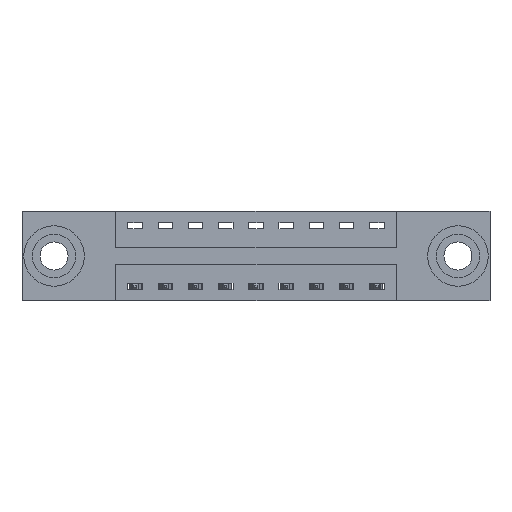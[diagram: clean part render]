
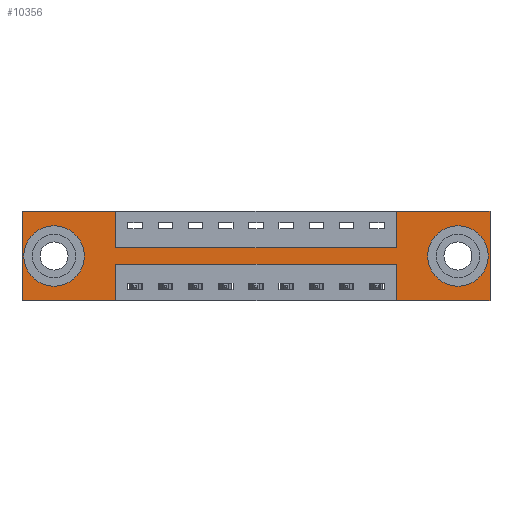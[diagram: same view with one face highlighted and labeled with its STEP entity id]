
A CAD part, front view. The second image highlights one B-rep face of the part: STEP entity #10356.
In plain terms, the highlighted planar face has unit normal (0, -1, 0).
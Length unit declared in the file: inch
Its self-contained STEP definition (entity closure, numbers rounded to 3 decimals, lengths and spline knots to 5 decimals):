
#183 = VERTEX_POINT ( 'NONE', #690 ) ;
#294 = DIRECTION ( 'NONE',  ( 0., -1., 0. ) ) ;
#352 = ORIENTED_EDGE ( 'NONE', *, *, #1826, .F. ) ;
#356 = CARTESIAN_POINT ( 'NONE',  ( 0.3875, 0., -0.22 ) ) ;
#470 = VERTEX_POINT ( 'NONE', #2785 ) ;
#529 = EDGE_CURVE ( 'NONE', #183, #3488, #4031, .T. ) ;
#548 = VECTOR ( 'NONE', #10347, 39.37008 ) ;
#568 = DIRECTION ( 'NONE',  ( 0., 0., -1. ) ) ;
#613 = DIRECTION ( 'NONE',  ( 0., 1., 0. ) ) ;
#633 = VECTOR ( 'NONE', #4701, 39.37008 ) ;
#659 = ORIENTED_EDGE ( 'NONE', *, *, #9545, .F. ) ;
#690 = CARTESIAN_POINT ( 'NONE',  ( 0., 0., -0.37 ) ) ;
#756 = ORIENTED_EDGE ( 'NONE', *, *, #10024, .T. ) ;
#826 = CARTESIAN_POINT ( 'NONE',  ( 0.3875, 0., -0.37 ) ) ;
#841 = LINE ( 'NONE', #9547, #9403 ) ;
#1276 = EDGE_LOOP ( 'NONE', ( #756, #8904 ) ) ;
#1315 = ORIENTED_EDGE ( 'NONE', *, *, #1736, .F. ) ;
#1346 = EDGE_CURVE ( 'NONE', #7675, #6904, #7158, .T. ) ;
#1589 = EDGE_CURVE ( 'NONE', #7468, #2087, #6758, .T. ) ;
#1601 = EDGE_CURVE ( 'NONE', #6904, #7675, #2371, .T. ) ;
#1736 = EDGE_CURVE ( 'NONE', #4805, #8246, #5458, .T. ) ;
#1826 = EDGE_CURVE ( 'NONE', #7963, #7468, #4422, .T. ) ;
#1853 = VERTEX_POINT ( 'NONE', #5337 ) ;
#1908 = FACE_OUTER_BOUND ( 'NONE', #7439, .T. ) ;
#1966 = EDGE_CURVE ( 'NONE', #9443, #183, #4812, .T. ) ;
#2033 = CARTESIAN_POINT ( 'NONE',  ( 0., 0., 0. ) ) ;
#2086 = AXIS2_PLACEMENT_3D ( 'NONE', #5556, #613, #6384 ) ;
#2087 = VERTEX_POINT ( 'NONE', #2345 ) ;
#2157 = ORIENTED_EDGE ( 'NONE', *, *, #1601, .T. ) ;
#2175 = FACE_BOUND ( 'NONE', #1276, .T. ) ;
#2242 = DIRECTION ( 'NONE',  ( 0., 1., 0. ) ) ;
#2345 = CARTESIAN_POINT ( 'NONE',  ( 1.5475, 0., -0.15 ) ) ;
#2371 = CIRCLE ( 'NONE', #2840, 0.078 ) ;
#2435 = ORIENTED_EDGE ( 'NONE', *, *, #1966, .F. ) ;
#2446 = ORIENTED_EDGE ( 'NONE', *, *, #3719, .F. ) ;
#2453 = CIRCLE ( 'NONE', #2086, 0.078 ) ;
#2479 = VECTOR ( 'NONE', #2958, 39.37008 ) ;
#2575 = LINE ( 'NONE', #9696, #633 ) ;
#2686 = DIRECTION ( 'NONE',  ( -1., 0., 0. ) ) ;
#2741 = LINE ( 'NONE', #2033, #548 ) ;
#2785 = CARTESIAN_POINT ( 'NONE',  ( 0.1325, 0., -0.107 ) ) ;
#2794 = ORIENTED_EDGE ( 'NONE', *, *, #1346, .T. ) ;
#2839 = CIRCLE ( 'NONE', #4439, 0.078 ) ;
#2840 = AXIS2_PLACEMENT_3D ( 'NONE', #8331, #3364, #9162 ) ;
#2868 = CARTESIAN_POINT ( 'NONE',  ( 0.3875, 0., -0.37 ) ) ;
#2958 = DIRECTION ( 'NONE',  ( 0., 0., 1. ) ) ;
#3050 = AXIS2_PLACEMENT_3D ( 'NONE', #10497, #5500, #568 ) ;
#3111 = VECTOR ( 'NONE', #4942, 39.37008 ) ;
#3279 = EDGE_CURVE ( 'NONE', #8254, #9443, #3356, .T. ) ;
#3356 = LINE ( 'NONE', #826, #3111 ) ;
#3364 = DIRECTION ( 'NONE',  ( 0., 1., 0. ) ) ;
#3365 = EDGE_LOOP ( 'NONE', ( #2794, #2157 ) ) ;
#3488 = VERTEX_POINT ( 'NONE', #6886 ) ;
#3719 = EDGE_CURVE ( 'NONE', #8246, #10174, #2575, .T. ) ;
#3782 = CARTESIAN_POINT ( 'NONE',  ( 0.3875, 0., -0.22 ) ) ;
#3908 = DIRECTION ( 'NONE',  ( 1., 0., 0. ) ) ;
#4031 = LINE ( 'NONE', #5329, #5977 ) ;
#4156 = CARTESIAN_POINT ( 'NONE',  ( 0.3875, 0., -0.15 ) ) ;
#4177 = CARTESIAN_POINT ( 'NONE',  ( 1.5475, 0., -0.22 ) ) ;
#4396 = EDGE_CURVE ( 'NONE', #6181, #470, #2453, .T. ) ;
#4402 = LINE ( 'NONE', #7893, #2479 ) ;
#4422 = LINE ( 'NONE', #6139, #6368 ) ;
#4439 = AXIS2_PLACEMENT_3D ( 'NONE', #7193, #2242, #8036 ) ;
#4473 = DIRECTION ( 'NONE',  ( 0., 0., 1. ) ) ;
#4694 = CARTESIAN_POINT ( 'NONE',  ( 0., 0., -0.37 ) ) ;
#4701 = DIRECTION ( 'NONE',  ( 0., 0., 1. ) ) ;
#4805 = VERTEX_POINT ( 'NONE', #9493 ) ;
#4812 = LINE ( 'NONE', #4694, #8969 ) ;
#4942 = DIRECTION ( 'NONE',  ( 0., 0., -1. ) ) ;
#4962 = CARTESIAN_POINT ( 'NONE',  ( 0.3875, 0., 0. ) ) ;
#5069 = VECTOR ( 'NONE', #9977, 39.37008 ) ;
#5329 = CARTESIAN_POINT ( 'NONE',  ( 0., 0., 0. ) ) ;
#5337 = CARTESIAN_POINT ( 'NONE',  ( 1.935, 0., 0. ) ) ;
#5383 = DIRECTION ( 'NONE',  ( 0., 0., -1. ) ) ;
#5458 = LINE ( 'NONE', #8461, #7407 ) ;
#5500 = DIRECTION ( 'NONE',  ( 0., 1., 0. ) ) ;
#5556 = CARTESIAN_POINT ( 'NONE',  ( 0.1325, 0., -0.185 ) ) ;
#5614 = VECTOR ( 'NONE', #3908, 39.37008 ) ;
#5777 = ORIENTED_EDGE ( 'NONE', *, *, #529, .F. ) ;
#5977 = VECTOR ( 'NONE', #4473, 39.37008 ) ;
#6012 = CARTESIAN_POINT ( 'NONE',  ( 1.5475, 0., -0.37 ) ) ;
#6058 = DIRECTION ( 'NONE',  ( 0., 0., -1. ) ) ;
#6139 = CARTESIAN_POINT ( 'NONE',  ( 0.3875, 0., 0. ) ) ;
#6140 = ORIENTED_EDGE ( 'NONE', *, *, #1589, .F. ) ;
#6181 = VERTEX_POINT ( 'NONE', #9931 ) ;
#6314 = FACE_BOUND ( 'NONE', #3365, .T. ) ;
#6368 = VECTOR ( 'NONE', #9467, 39.37008 ) ;
#6384 = DIRECTION ( 'NONE',  ( 0., 0., 1. ) ) ;
#6397 = ORIENTED_EDGE ( 'NONE', *, *, #8876, .F. ) ;
#6403 = ORIENTED_EDGE ( 'NONE', *, *, #7088, .F. ) ;
#6758 = LINE ( 'NONE', #4156, #5069 ) ;
#6886 = CARTESIAN_POINT ( 'NONE',  ( 0., 0., 0. ) ) ;
#6904 = VERTEX_POINT ( 'NONE', #9511 ) ;
#6933 = EDGE_CURVE ( 'NONE', #1853, #4805, #841, .T. ) ;
#6979 = VECTOR ( 'NONE', #8749, 39.37008 ) ;
#7088 = EDGE_CURVE ( 'NONE', #3488, #7963, #10315, .T. ) ;
#7158 = CIRCLE ( 'NONE', #3050, 0.078 ) ;
#7193 = CARTESIAN_POINT ( 'NONE',  ( 0.1325, 0., -0.185 ) ) ;
#7252 = ORIENTED_EDGE ( 'NONE', *, *, #3279, .F. ) ;
#7407 = VECTOR ( 'NONE', #2686, 39.37008 ) ;
#7439 = EDGE_LOOP ( 'NONE', ( #7252, #659, #2446, #1315, #8600, #10509, #6397, #6140, #352, #6403, #5777, #2435 ) ) ;
#7468 = VERTEX_POINT ( 'NONE', #7662 ) ;
#7662 = CARTESIAN_POINT ( 'NONE',  ( 0.3875, 0., -0.15 ) ) ;
#7675 = VERTEX_POINT ( 'NONE', #9646 ) ;
#7679 = CARTESIAN_POINT ( 'NONE',  ( 0., 0., -0.37 ) ) ;
#7893 = CARTESIAN_POINT ( 'NONE',  ( 1.5475, 0., 0. ) ) ;
#7963 = VERTEX_POINT ( 'NONE', #4962 ) ;
#8036 = DIRECTION ( 'NONE',  ( 0., 0., 1. ) ) ;
#8045 = CARTESIAN_POINT ( 'NONE',  ( 0., 0., 0. ) ) ;
#8113 = CARTESIAN_POINT ( 'NONE',  ( 1.5475, 0., 0. ) ) ;
#8246 = VERTEX_POINT ( 'NONE', #6012 ) ;
#8254 = VERTEX_POINT ( 'NONE', #356 ) ;
#8331 = CARTESIAN_POINT ( 'NONE',  ( 1.8025, 0., -0.185 ) ) ;
#8461 = CARTESIAN_POINT ( 'NONE',  ( 0., 0., -0.37 ) ) ;
#8600 = ORIENTED_EDGE ( 'NONE', *, *, #6933, .F. ) ;
#8684 = AXIS2_PLACEMENT_3D ( 'NONE', #7679, #294, #6058 ) ;
#8749 = DIRECTION ( 'NONE',  ( -1., 0., 0. ) ) ;
#8832 = EDGE_CURVE ( 'NONE', #9062, #1853, #2741, .T. ) ;
#8835 = DIRECTION ( 'NONE',  ( -1., 0., 0. ) ) ;
#8876 = EDGE_CURVE ( 'NONE', #2087, #9062, #4402, .T. ) ;
#8904 = ORIENTED_EDGE ( 'NONE', *, *, #4396, .T. ) ;
#8969 = VECTOR ( 'NONE', #8835, 39.37008 ) ;
#9062 = VERTEX_POINT ( 'NONE', #8113 ) ;
#9162 = DIRECTION ( 'NONE',  ( 0., 0., -1. ) ) ;
#9197 = LINE ( 'NONE', #3782, #6979 ) ;
#9403 = VECTOR ( 'NONE', #5383, 39.37008 ) ;
#9443 = VERTEX_POINT ( 'NONE', #2868 ) ;
#9467 = DIRECTION ( 'NONE',  ( 0., 0., -1. ) ) ;
#9493 = CARTESIAN_POINT ( 'NONE',  ( 1.935, 0., -0.37 ) ) ;
#9511 = CARTESIAN_POINT ( 'NONE',  ( 1.8025, 0., -0.263 ) ) ;
#9545 = EDGE_CURVE ( 'NONE', #10174, #8254, #9197, .T. ) ;
#9547 = CARTESIAN_POINT ( 'NONE',  ( 1.935, 0., 0. ) ) ;
#9646 = CARTESIAN_POINT ( 'NONE',  ( 1.8025, 0., -0.107 ) ) ;
#9696 = CARTESIAN_POINT ( 'NONE',  ( 1.5475, 0., -0.37 ) ) ;
#9931 = CARTESIAN_POINT ( 'NONE',  ( 0.1325, 0., -0.263 ) ) ;
#9977 = DIRECTION ( 'NONE',  ( 1., 0., 0. ) ) ;
#10024 = EDGE_CURVE ( 'NONE', #470, #6181, #2839, .T. ) ;
#10174 = VERTEX_POINT ( 'NONE', #4177 ) ;
#10215 = PLANE ( 'NONE',  #8684 ) ;
#10315 = LINE ( 'NONE', #8045, #5614 ) ;
#10347 = DIRECTION ( 'NONE',  ( 1., 0., 0. ) ) ;
#10356 = ADVANCED_FACE ( 'NONE', ( #6314, #2175, #1908 ), #10215, .T. ) ;
#10497 = CARTESIAN_POINT ( 'NONE',  ( 1.8025, 0., -0.185 ) ) ;
#10509 = ORIENTED_EDGE ( 'NONE', *, *, #8832, .F. ) ;
